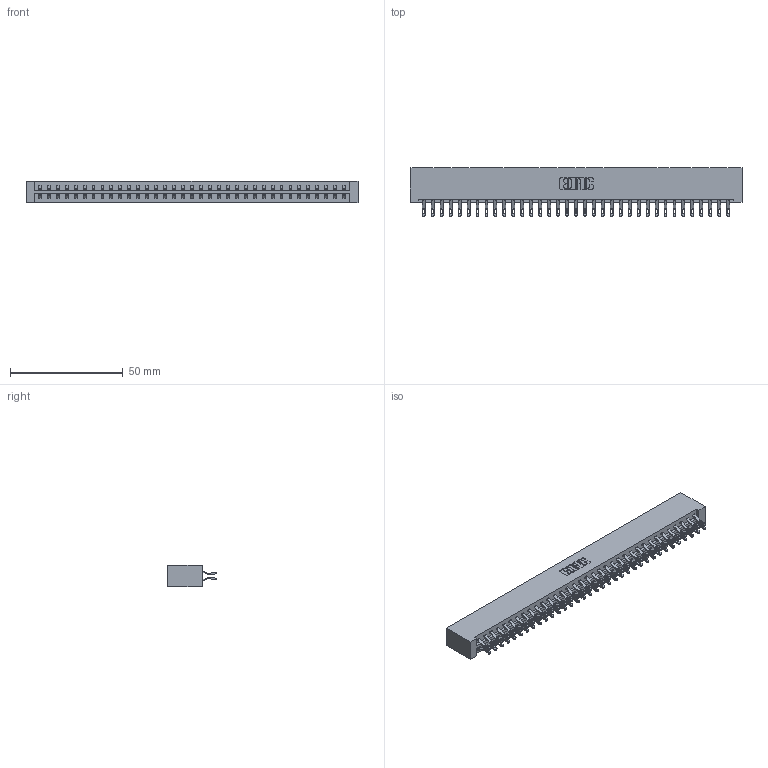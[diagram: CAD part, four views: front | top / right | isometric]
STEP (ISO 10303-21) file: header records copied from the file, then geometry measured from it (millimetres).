
FILE_DESCRIPTION (( 'STEP AP203' ), '1' );
FILE_NAME ('833-070-555-201.STEP', '2020-06-05T12:50:18', ( '' ), ( '' ), 'SwSTEP 2.0', 'SolidWorks 2020', '' );
FILE_SCHEMA (( 'CONFIG_CONTROL_DESIGN' ));
Length unit declared in the file: inch
Products named in the file (3): 833 Part_Lugless; 833-070-555-201; 345-292-001_555 Tail
Assembly tree (71 placements, depth 2):
  833-070-555-201
    833 Part_Lugless
    345-292-001_555 Tail  x70
Bounding box: 146.94 x 21.47 x 9.4 mm (x, y, z)
Volume: 15771.4 mm3; surface area: 19354.2 mm2
Topology: 71 solids, 71 shells, 4166 faces, 13097 edges, 8730 vertices
Faces by surface type: plane 2446, cylinder 1720
Entity records: 23471 total; most frequent: CARTESIAN_POINT 3932, ORIENTED_EDGE 3838, DIRECTION 3335, EDGE_CURVE 1919, LINE 1779, VECTOR 1779, VERTEX_POINT 1278, AXIS2_PLACEMENT_3D 778
